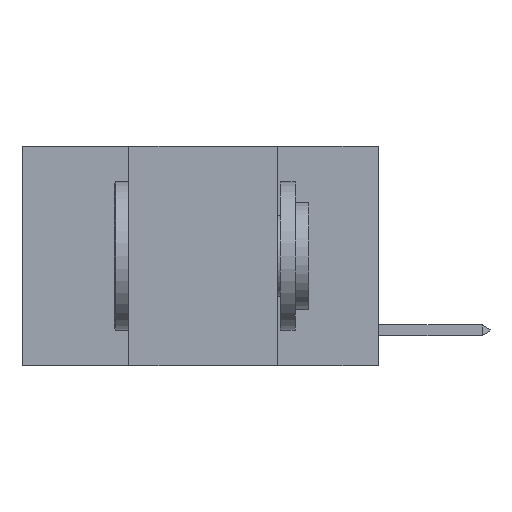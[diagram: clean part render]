
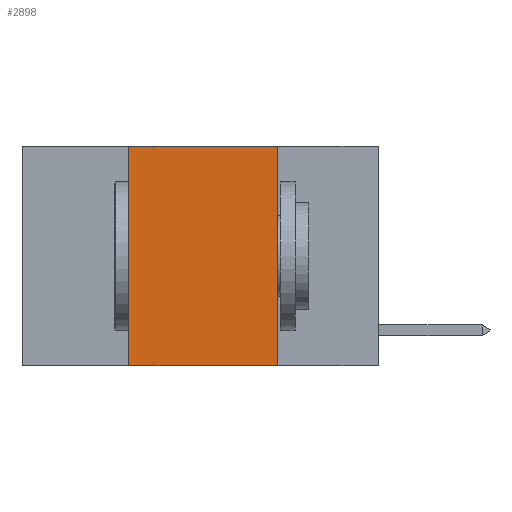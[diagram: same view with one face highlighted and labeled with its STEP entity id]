
A CAD part, left-side view. The second image highlights one B-rep face of the part: STEP entity #2898.
In plain terms, the highlighted planar face has unit normal (-1, 0, 0).
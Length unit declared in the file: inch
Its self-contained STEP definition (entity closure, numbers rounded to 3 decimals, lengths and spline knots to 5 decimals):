
#116 = VERTEX_POINT ( 'NONE', #8487 ) ;
#203 = CARTESIAN_POINT ( 'NONE',  ( 0., 0.6, -0.37 ) ) ;
#293 = EDGE_CURVE ( 'NONE', #6220, #11320, #1225, .T. ) ;
#1040 = VECTOR ( 'NONE', #3091, 39.37008 ) ;
#1225 = LINE ( 'NONE', #5604, #6847 ) ;
#2361 = ORIENTED_EDGE ( 'NONE', *, *, #6191, .F. ) ;
#2440 = DIRECTION ( 'NONE',  ( 0., 0., 1. ) ) ;
#2898 = ADVANCED_FACE ( 'NONE', ( #12920 ), #9601, .F. ) ;
#3091 = DIRECTION ( 'NONE',  ( 0., 0., -1. ) ) ;
#3598 = CARTESIAN_POINT ( 'NONE',  ( 0., 0.42, 0. ) ) ;
#4381 = CARTESIAN_POINT ( 'NONE',  ( 0., 0.17, 0. ) ) ;
#4533 = DIRECTION ( 'NONE',  ( 0., -1., 0. ) ) ;
#4746 = CARTESIAN_POINT ( 'NONE',  ( 0., 0.42, 0. ) ) ;
#5040 = ORIENTED_EDGE ( 'NONE', *, *, #6228, .T. ) ;
#5604 = CARTESIAN_POINT ( 'NONE',  ( 0., 0.6, 0. ) ) ;
#5747 = DIRECTION ( 'NONE',  ( 0., -1., 0. ) ) ;
#6191 = EDGE_CURVE ( 'NONE', #116, #6220, #13633, .T. ) ;
#6220 = VERTEX_POINT ( 'NONE', #4746 ) ;
#6228 = EDGE_CURVE ( 'NONE', #116, #10722, #12457, .T. ) ;
#6333 = DIRECTION ( 'NONE',  ( 1., 0., 0. ) ) ;
#6847 = VECTOR ( 'NONE', #4533, 39.37008 ) ;
#7336 = CARTESIAN_POINT ( 'NONE',  ( 0., 0.17, -0.37 ) ) ;
#7355 = ORIENTED_EDGE ( 'NONE', *, *, #11336, .F. ) ;
#7816 = VECTOR ( 'NONE', #5747, 39.37008 ) ;
#8487 = CARTESIAN_POINT ( 'NONE',  ( 0., 0.42, -0.37 ) ) ;
#8580 = DIRECTION ( 'NONE',  ( 0., 0., -1. ) ) ;
#9448 = CARTESIAN_POINT ( 'NONE',  ( 0., 0.6, 0. ) ) ;
#9601 = PLANE ( 'NONE',  #11269 ) ;
#10374 = VECTOR ( 'NONE', #2440, 39.37008 ) ;
#10447 = EDGE_LOOP ( 'NONE', ( #7355, #14176, #2361, #5040 ) ) ;
#10722 = VERTEX_POINT ( 'NONE', #7336 ) ;
#11269 = AXIS2_PLACEMENT_3D ( 'NONE', #9448, #6333, #8580 ) ;
#11320 = VERTEX_POINT ( 'NONE', #12969 ) ;
#11336 = EDGE_CURVE ( 'NONE', #11320, #10722, #11943, .T. ) ;
#11943 = LINE ( 'NONE', #4381, #1040 ) ;
#12457 = LINE ( 'NONE', #203, #7816 ) ;
#12920 = FACE_OUTER_BOUND ( 'NONE', #10447, .T. ) ;
#12969 = CARTESIAN_POINT ( 'NONE',  ( 0., 0.17, 0. ) ) ;
#13633 = LINE ( 'NONE', #3598, #10374 ) ;
#14176 = ORIENTED_EDGE ( 'NONE', *, *, #293, .F. ) ;
